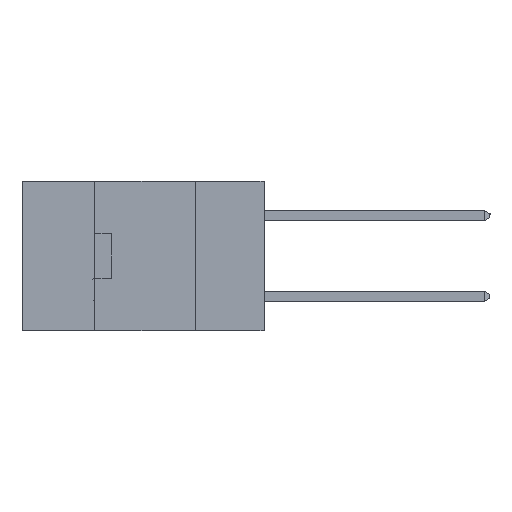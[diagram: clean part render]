
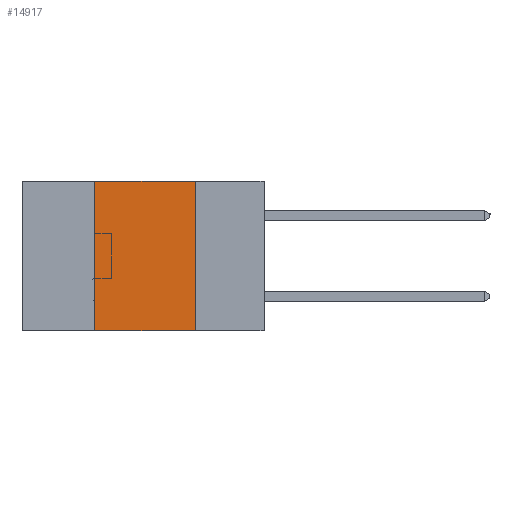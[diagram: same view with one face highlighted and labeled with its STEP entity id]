
A CAD part, left-side view. The second image highlights one B-rep face of the part: STEP entity #14917.
In plain terms, the highlighted planar face has unit normal (-1, 0, 0).
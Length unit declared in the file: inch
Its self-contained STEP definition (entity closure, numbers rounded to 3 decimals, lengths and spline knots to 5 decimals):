
#73 = EDGE_CURVE ( 'NONE', #28206, #19626, #23036, .T. ) ;
#889 = DIRECTION ( 'NONE',  ( 1., 0., 0. ) ) ;
#1036 = FACE_OUTER_BOUND ( 'NONE', #19702, .T. ) ;
#1397 = ORIENTED_EDGE ( 'NONE', *, *, #19589, .F. ) ;
#2960 = CARTESIAN_POINT ( 'NONE',  ( 0., 0.6, 0. ) ) ;
#3107 = LINE ( 'NONE', #2960, #4052 ) ;
#3366 = CARTESIAN_POINT ( 'NONE',  ( 0., 0.42, -0.37 ) ) ;
#4052 = VECTOR ( 'NONE', #15831, 39.37008 ) ;
#4409 = VECTOR ( 'NONE', #14243, 39.37008 ) ;
#4830 = PLANE ( 'NONE',  #27243 ) ;
#5848 = LINE ( 'NONE', #3366, #19307 ) ;
#7760 = ORIENTED_EDGE ( 'NONE', *, *, #15205, .F. ) ;
#9225 = CARTESIAN_POINT ( 'NONE',  ( 0., 0.17, -0.37 ) ) ;
#13885 = VECTOR ( 'NONE', #28391, 39.37008 ) ;
#14243 = DIRECTION ( 'NONE',  ( 0., 0., -1. ) ) ;
#14917 = ADVANCED_FACE ( 'NONE', ( #1036 ), #4830, .F. ) ;
#15205 = EDGE_CURVE ( 'NONE', #26274, #27814, #5848, .T. ) ;
#15831 = DIRECTION ( 'NONE',  ( 0., -1., 0. ) ) ;
#16677 = CARTESIAN_POINT ( 'NONE',  ( 0., 0.42, 0. ) ) ;
#19144 = LINE ( 'NONE', #21646, #13885 ) ;
#19307 = VECTOR ( 'NONE', #23723, 39.37008 ) ;
#19589 = EDGE_CURVE ( 'NONE', #27814, #28206, #3107, .T. ) ;
#19626 = VERTEX_POINT ( 'NONE', #9225 ) ;
#19702 = EDGE_LOOP ( 'NONE', ( #28441, #1397, #7760, #23703 ) ) ;
#21646 = CARTESIAN_POINT ( 'NONE',  ( 0., 0.6, -0.37 ) ) ;
#22693 = DIRECTION ( 'NONE',  ( 0., 0., -1. ) ) ;
#23036 = LINE ( 'NONE', #23478, #4409 ) ;
#23478 = CARTESIAN_POINT ( 'NONE',  ( 0., 0.17, -0.37 ) ) ;
#23703 = ORIENTED_EDGE ( 'NONE', *, *, #28419, .T. ) ;
#23723 = DIRECTION ( 'NONE',  ( 0., 0., 1. ) ) ;
#24907 = CARTESIAN_POINT ( 'NONE',  ( 0., 0.42, -0.37 ) ) ;
#25444 = CARTESIAN_POINT ( 'NONE',  ( 0., 0.17, 0. ) ) ;
#25474 = CARTESIAN_POINT ( 'NONE',  ( 0., 0.6, 0. ) ) ;
#26274 = VERTEX_POINT ( 'NONE', #24907 ) ;
#27243 = AXIS2_PLACEMENT_3D ( 'NONE', #25474, #889, #22693 ) ;
#27814 = VERTEX_POINT ( 'NONE', #16677 ) ;
#28206 = VERTEX_POINT ( 'NONE', #25444 ) ;
#28391 = DIRECTION ( 'NONE',  ( 0., -1., 0. ) ) ;
#28419 = EDGE_CURVE ( 'NONE', #26274, #19626, #19144, .T. ) ;
#28441 = ORIENTED_EDGE ( 'NONE', *, *, #73, .F. ) ;
